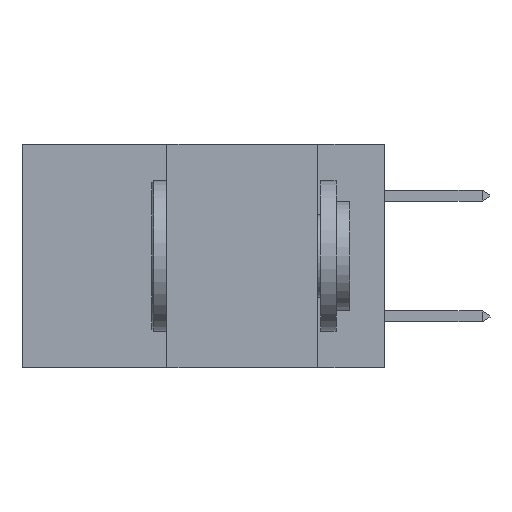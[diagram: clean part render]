
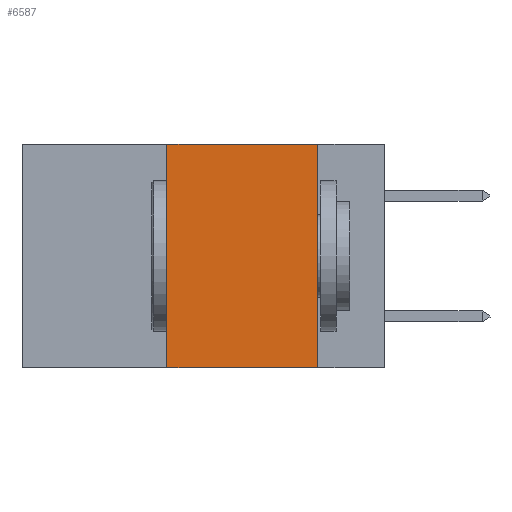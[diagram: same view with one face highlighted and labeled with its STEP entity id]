
A CAD part, left-side view. The second image highlights one B-rep face of the part: STEP entity #6587.
In plain terms, the highlighted planar face has unit normal (-1, 0, 0).
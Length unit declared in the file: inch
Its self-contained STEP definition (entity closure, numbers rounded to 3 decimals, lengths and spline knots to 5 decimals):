
#1396 = LINE ( 'NONE', #5632, #16314 ) ;
#2105 = CARTESIAN_POINT ( 'NONE',  ( 0., 0.6, 0. ) ) ;
#2167 = DIRECTION ( 'NONE',  ( 0., 0., -1. ) ) ;
#2757 = EDGE_CURVE ( 'NONE', #20760, #4588, #5312, .T. ) ;
#3252 = CARTESIAN_POINT ( 'NONE',  ( 0., 0.36, 0. ) ) ;
#4456 = CARTESIAN_POINT ( 'NONE',  ( 0., 0.11, 0. ) ) ;
#4588 = VERTEX_POINT ( 'NONE', #18543 ) ;
#4658 = CARTESIAN_POINT ( 'NONE',  ( 0., 0.11, 0. ) ) ;
#4691 = DIRECTION ( 'NONE',  ( 0., 0., -1. ) ) ;
#4993 = DIRECTION ( 'NONE',  ( 0., 0., 1. ) ) ;
#5312 = LINE ( 'NONE', #4658, #8643 ) ;
#5632 = CARTESIAN_POINT ( 'NONE',  ( 0., 0.6, -0.37 ) ) ;
#6587 = ADVANCED_FACE ( 'NONE', ( #10333 ), #18818, .F. ) ;
#6590 = EDGE_CURVE ( 'NONE', #6633, #4588, #1396, .T. ) ;
#6633 = VERTEX_POINT ( 'NONE', #10690 ) ;
#8007 = VECTOR ( 'NONE', #4993, 39.37008 ) ;
#8077 = DIRECTION ( 'NONE',  ( 0., -1., 0. ) ) ;
#8558 = LINE ( 'NONE', #3252, #8007 ) ;
#8643 = VECTOR ( 'NONE', #4691, 39.37008 ) ;
#10333 = FACE_OUTER_BOUND ( 'NONE', #17345, .T. ) ;
#10425 = VECTOR ( 'NONE', #8077, 39.37008 ) ;
#10690 = CARTESIAN_POINT ( 'NONE',  ( 0., 0.36, -0.37 ) ) ;
#11020 = AXIS2_PLACEMENT_3D ( 'NONE', #2105, #12203, #2167 ) ;
#11372 = ORIENTED_EDGE ( 'NONE', *, *, #2757, .F. ) ;
#12158 = ORIENTED_EDGE ( 'NONE', *, *, #6590, .T. ) ;
#12203 = DIRECTION ( 'NONE',  ( 1., 0., 0. ) ) ;
#12953 = EDGE_CURVE ( 'NONE', #18780, #20760, #18232, .T. ) ;
#14370 = EDGE_CURVE ( 'NONE', #6633, #18780, #8558, .T. ) ;
#14902 = ORIENTED_EDGE ( 'NONE', *, *, #14370, .F. ) ;
#16314 = VECTOR ( 'NONE', #17266, 39.37008 ) ;
#16590 = CARTESIAN_POINT ( 'NONE',  ( 0., 0.36, 0. ) ) ;
#17266 = DIRECTION ( 'NONE',  ( 0., -1., 0. ) ) ;
#17345 = EDGE_LOOP ( 'NONE', ( #11372, #19866, #14902, #12158 ) ) ;
#18232 = LINE ( 'NONE', #19701, #10425 ) ;
#18543 = CARTESIAN_POINT ( 'NONE',  ( 0., 0.11, -0.37 ) ) ;
#18780 = VERTEX_POINT ( 'NONE', #16590 ) ;
#18818 = PLANE ( 'NONE',  #11020 ) ;
#19701 = CARTESIAN_POINT ( 'NONE',  ( 0., 0.6, 0. ) ) ;
#19866 = ORIENTED_EDGE ( 'NONE', *, *, #12953, .F. ) ;
#20760 = VERTEX_POINT ( 'NONE', #4456 ) ;
